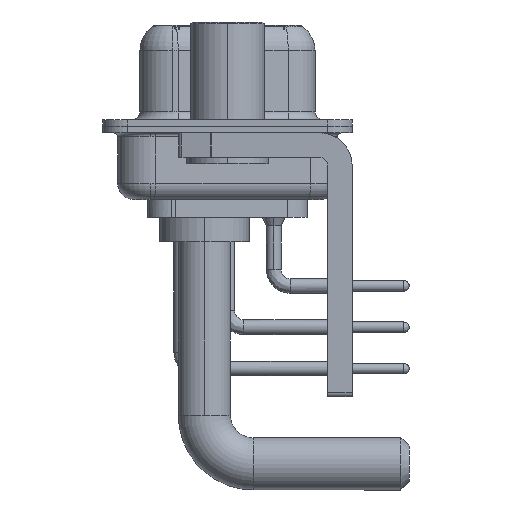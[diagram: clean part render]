
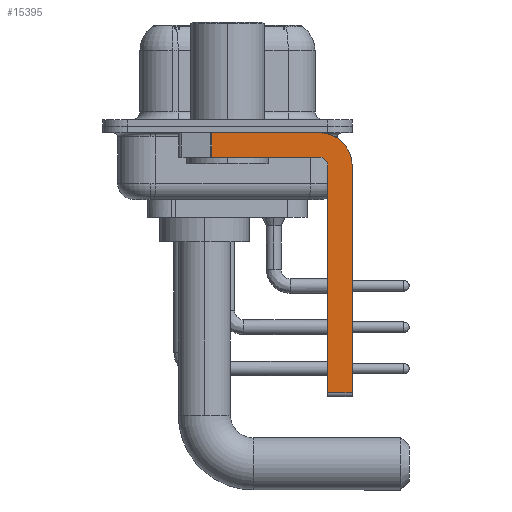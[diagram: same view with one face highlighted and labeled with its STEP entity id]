
A CAD part, left-side view. The second image highlights one B-rep face of the part: STEP entity #15395.
In plain terms, the highlighted planar face has unit normal (-1, 0, 0).
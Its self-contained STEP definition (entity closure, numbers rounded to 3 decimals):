
#429 = CARTESIAN_POINT ( 'NONE',  ( -2.9, -5.65, -2.4 ) ) ;
#601 = DIRECTION ( 'NONE',  ( 0., 0., 1. ) ) ;
#692 = DIRECTION ( 'NONE',  ( 0., 0., -1. ) ) ;
#910 = DIRECTION ( 'NONE',  ( 1., 0., 0. ) ) ;
#1507 = LINE ( 'NONE', #25309, #15013 ) ;
#2443 = ORIENTED_EDGE ( 'NONE', *, *, #4292, .F. ) ;
#2717 = CARTESIAN_POINT ( 'NONE',  ( -2.9, 0.978, -0.4 ) ) ;
#3322 = EDGE_CURVE ( 'NONE', #10839, #24238, #14044, .T. ) ;
#3734 = CARTESIAN_POINT ( 'NONE',  ( -2.9, -5.65, -1.9 ) ) ;
#4030 = DIRECTION ( 'NONE',  ( 1., 0., 0. ) ) ;
#4200 = DIRECTION ( 'NONE',  ( 0., 0., -1. ) ) ;
#4292 = EDGE_CURVE ( 'NONE', #19768, #15804, #6512, .T. ) ;
#5762 = EDGE_CURVE ( 'NONE', #27899, #26978, #21564, .T. ) ;
#6230 = AXIS2_PLACEMENT_3D ( 'NONE', #429, #33396, #601 ) ;
#6486 = DIRECTION ( 'NONE',  ( 0., 0., 1. ) ) ;
#6512 = CIRCLE ( 'NONE', #15079, 2. ) ;
#6963 = CARTESIAN_POINT ( 'NONE',  ( -2.9, -5.65, -16.35 ) ) ;
#7316 = EDGE_CURVE ( 'NONE', #26956, #27899, #1507, .T. ) ;
#7489 = ORIENTED_EDGE ( 'NONE', *, *, #9895, .F. ) ;
#7538 = CARTESIAN_POINT ( 'NONE',  ( -2.9, -6.15, -16.35 ) ) ;
#7958 = ORIENTED_EDGE ( 'NONE', *, *, #10618, .T. ) ;
#9097 = DIRECTION ( 'NONE',  ( 0., 1., 0. ) ) ;
#9895 = EDGE_CURVE ( 'NONE', #15804, #16378, #32070, .T. ) ;
#10618 = EDGE_CURVE ( 'NONE', #26956, #16378, #31947, .T. ) ;
#10839 = VERTEX_POINT ( 'NONE', #2717 ) ;
#11967 = ORIENTED_EDGE ( 'NONE', *, *, #28558, .F. ) ;
#12009 = CARTESIAN_POINT ( 'NONE',  ( -2.9, -5.65, -0.4 ) ) ;
#12545 = EDGE_CURVE ( 'NONE', #10839, #19768, #18837, .T. ) ;
#13922 = VECTOR ( 'NONE', #26772, 1000. ) ;
#14044 = LINE ( 'NONE', #24655, #32583 ) ;
#14097 = CARTESIAN_POINT ( 'NONE',  ( -2.9, -5.65, -2.4 ) ) ;
#14552 = FACE_OUTER_BOUND ( 'NONE', #20295, .T. ) ;
#15013 = VECTOR ( 'NONE', #6486, 1000. ) ;
#15079 = AXIS2_PLACEMENT_3D ( 'NONE', #14097, #910, #27860 ) ;
#15099 = ORIENTED_EDGE ( 'NONE', *, *, #7316, .F. ) ;
#15209 = VECTOR ( 'NONE', #16187, 1000. ) ;
#15395 = ADVANCED_FACE ( 'NONE', ( #14552 ), #25856, .F. ) ;
#15504 = CARTESIAN_POINT ( 'NONE',  ( -2.9, 0.978, -1.9 ) ) ;
#15804 = VERTEX_POINT ( 'NONE', #22312 ) ;
#16187 = DIRECTION ( 'NONE',  ( 0., -1., 0. ) ) ;
#16378 = VERTEX_POINT ( 'NONE', #28589 ) ;
#16637 = CARTESIAN_POINT ( 'NONE',  ( -2.9, -6.15, -2.4 ) ) ;
#18837 = LINE ( 'NONE', #24653, #15209 ) ;
#19639 = VECTOR ( 'NONE', #26126, 1000. ) ;
#19768 = VERTEX_POINT ( 'NONE', #12009 ) ;
#20041 = CARTESIAN_POINT ( 'NONE',  ( -2.9, -5.65, -2.4 ) ) ;
#20295 = EDGE_LOOP ( 'NONE', ( #22580, #34185, #11967, #29178, #15099, #7958, #7489, #2443 ) ) ;
#20950 = AXIS2_PLACEMENT_3D ( 'NONE', #20041, #4030, #4200 ) ;
#21564 = CIRCLE ( 'NONE', #6230, 0.5 ) ;
#22312 = CARTESIAN_POINT ( 'NONE',  ( -2.9, -7.65, -2.4 ) ) ;
#22580 = ORIENTED_EDGE ( 'NONE', *, *, #12545, .F. ) ;
#24238 = VERTEX_POINT ( 'NONE', #15504 ) ;
#24653 = CARTESIAN_POINT ( 'NONE',  ( -2.9, 3., -0.4 ) ) ;
#24655 = CARTESIAN_POINT ( 'NONE',  ( -2.9, 0.978, -1.9 ) ) ;
#25309 = CARTESIAN_POINT ( 'NONE',  ( -2.9, -6.15, -16.6 ) ) ;
#25856 = PLANE ( 'NONE',  #20950 ) ;
#26126 = DIRECTION ( 'NONE',  ( 0., -1., 0. ) ) ;
#26772 = DIRECTION ( 'NONE',  ( 0., 0., -1. ) ) ;
#26956 = VERTEX_POINT ( 'NONE', #7538 ) ;
#26978 = VERTEX_POINT ( 'NONE', #31457 ) ;
#27616 = VECTOR ( 'NONE', #9097, 1000. ) ;
#27860 = DIRECTION ( 'NONE',  ( 0., 0., -1. ) ) ;
#27899 = VERTEX_POINT ( 'NONE', #16637 ) ;
#28558 = EDGE_CURVE ( 'NONE', #26978, #24238, #30520, .T. ) ;
#28589 = CARTESIAN_POINT ( 'NONE',  ( -2.9, -7.65, -16.35 ) ) ;
#29178 = ORIENTED_EDGE ( 'NONE', *, *, #5762, .F. ) ;
#30520 = LINE ( 'NONE', #3734, #27616 ) ;
#31457 = CARTESIAN_POINT ( 'NONE',  ( -2.9, -5.65, -1.9 ) ) ;
#31947 = LINE ( 'NONE', #6963, #19639 ) ;
#32070 = LINE ( 'NONE', #32591, #13922 ) ;
#32583 = VECTOR ( 'NONE', #692, 1000. ) ;
#32591 = CARTESIAN_POINT ( 'NONE',  ( -2.9, -7.65, -2.4 ) ) ;
#33396 = DIRECTION ( 'NONE',  ( -1., 0., 0. ) ) ;
#34185 = ORIENTED_EDGE ( 'NONE', *, *, #3322, .T. ) ;
